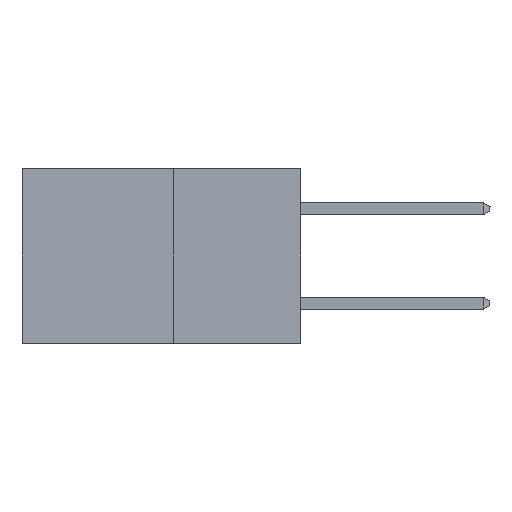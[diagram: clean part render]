
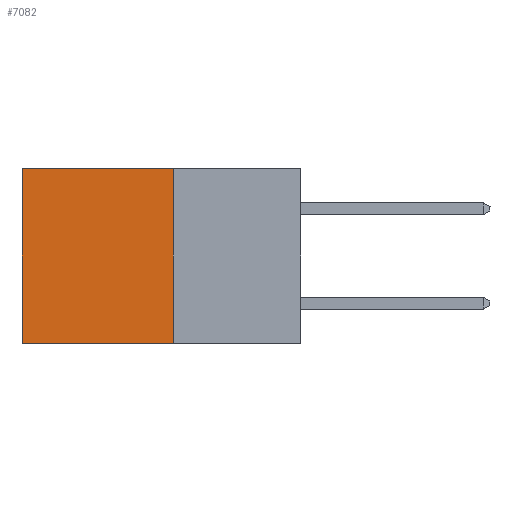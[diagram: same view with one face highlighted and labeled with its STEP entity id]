
A CAD part, left-side view. The second image highlights one B-rep face of the part: STEP entity #7082.
In plain terms, the highlighted planar face has unit normal (-1, 0, 0).
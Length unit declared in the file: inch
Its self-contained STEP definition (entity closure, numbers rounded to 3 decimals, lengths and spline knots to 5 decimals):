
#33 = CARTESIAN_POINT ( 'NONE',  ( 0.277, 0.27, 0. ) ) ;
#249 = VERTEX_POINT ( 'NONE', #2007 ) ;
#443 = LINE ( 'NONE', #1968, #6316 ) ;
#655 = LINE ( 'NONE', #2389, #4588 ) ;
#1008 = EDGE_CURVE ( 'NONE', #3942, #249, #4016, .T. ) ;
#1344 = CARTESIAN_POINT ( 'NONE',  ( 0.277, 0.59, -0.37 ) ) ;
#1484 = EDGE_CURVE ( 'NONE', #3942, #6138, #655, .T. ) ;
#1712 = EDGE_CURVE ( 'NONE', #249, #8225, #443, .T. ) ;
#1968 = CARTESIAN_POINT ( 'NONE',  ( 0.277, 0.27, -0.37 ) ) ;
#2007 = CARTESIAN_POINT ( 'NONE',  ( 0.277, 0.27, -0.37 ) ) ;
#2026 = VECTOR ( 'NONE', #4038, 39.37008 ) ;
#2070 = DIRECTION ( 'NONE',  ( 0., 1., 0. ) ) ;
#2389 = CARTESIAN_POINT ( 'NONE',  ( 0.277, 0.27, 0. ) ) ;
#2408 = AXIS2_PLACEMENT_3D ( 'NONE', #7373, #3038, #8112 ) ;
#2563 = EDGE_LOOP ( 'NONE', ( #3361, #3272, #4338, #4632 ) ) ;
#2681 = CARTESIAN_POINT ( 'NONE',  ( 0.277, 0.59, -0.37 ) ) ;
#2936 = DIRECTION ( 'NONE',  ( 0., 0., -1. ) ) ;
#3038 = DIRECTION ( 'NONE',  ( 1., 0., 0. ) ) ;
#3272 = ORIENTED_EDGE ( 'NONE', *, *, #1712, .F. ) ;
#3361 = ORIENTED_EDGE ( 'NONE', *, *, #5683, .T. ) ;
#3942 = VERTEX_POINT ( 'NONE', #33 ) ;
#3967 = CARTESIAN_POINT ( 'NONE',  ( 0.277, 0.27, -0.37 ) ) ;
#4016 = LINE ( 'NONE', #3967, #2026 ) ;
#4038 = DIRECTION ( 'NONE',  ( 0., 0., -1. ) ) ;
#4338 = ORIENTED_EDGE ( 'NONE', *, *, #1008, .F. ) ;
#4588 = VECTOR ( 'NONE', #8118, 39.37008 ) ;
#4632 = ORIENTED_EDGE ( 'NONE', *, *, #1484, .T. ) ;
#4716 = CARTESIAN_POINT ( 'NONE',  ( 0.277, 0.59, 0. ) ) ;
#5222 = PLANE ( 'NONE',  #2408 ) ;
#5674 = FACE_OUTER_BOUND ( 'NONE', #2563, .T. ) ;
#5683 = EDGE_CURVE ( 'NONE', #6138, #8225, #9016, .T. ) ;
#6138 = VERTEX_POINT ( 'NONE', #4716 ) ;
#6316 = VECTOR ( 'NONE', #2070, 39.37008 ) ;
#7082 = ADVANCED_FACE ( 'NONE', ( #5674 ), #5222, .F. ) ;
#7124 = VECTOR ( 'NONE', #2936, 39.37008 ) ;
#7373 = CARTESIAN_POINT ( 'NONE',  ( 0.277, 0.27, -0.37 ) ) ;
#8112 = DIRECTION ( 'NONE',  ( 0., 0., -1. ) ) ;
#8118 = DIRECTION ( 'NONE',  ( 0., 1., 0. ) ) ;
#8225 = VERTEX_POINT ( 'NONE', #2681 ) ;
#9016 = LINE ( 'NONE', #1344, #7124 ) ;
